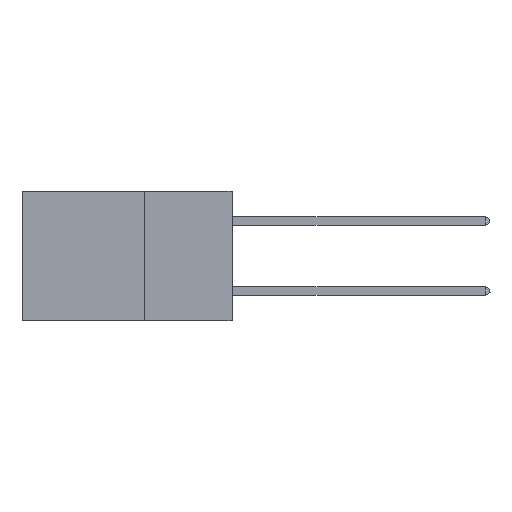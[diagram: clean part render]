
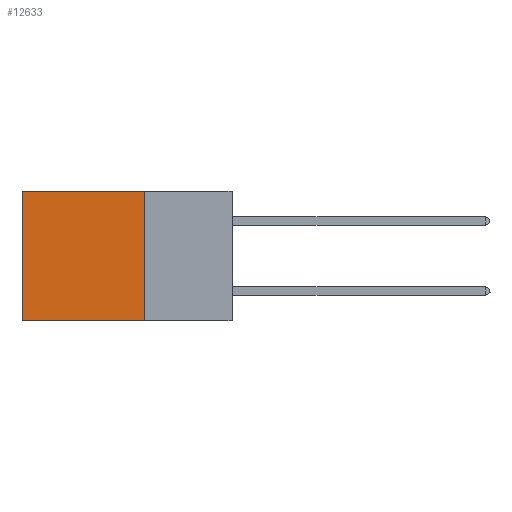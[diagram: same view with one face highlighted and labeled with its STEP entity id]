
A CAD part, left-side view. The second image highlights one B-rep face of the part: STEP entity #12633.
In plain terms, the highlighted planar face has unit normal (-1, 0, 0).
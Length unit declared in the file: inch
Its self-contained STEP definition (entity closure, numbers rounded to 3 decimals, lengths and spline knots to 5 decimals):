
#1057 = CARTESIAN_POINT ( 'NONE',  ( 0.2875, 0.25, 0. ) ) ;
#1160 = CARTESIAN_POINT ( 'NONE',  ( 0.2875, 0.6, -0.37 ) ) ;
#1495 = PLANE ( 'NONE',  #9630 ) ;
#3088 = CARTESIAN_POINT ( 'NONE',  ( 0.2875, 0.25, 0. ) ) ;
#3526 = CARTESIAN_POINT ( 'NONE',  ( 0.2875, 0.25, 0. ) ) ;
#3814 = CARTESIAN_POINT ( 'NONE',  ( 0.2875, 0.25, -0.37 ) ) ;
#4068 = VECTOR ( 'NONE', #19564, 39.37008 ) ;
#5462 = DIRECTION ( 'NONE',  ( 1., 0., 0. ) ) ;
#5641 = ORIENTED_EDGE ( 'NONE', *, *, #22986, .F. ) ;
#5736 = LINE ( 'NONE', #3814, #12072 ) ;
#8291 = CARTESIAN_POINT ( 'NONE',  ( 0.2875, 0.6, 0. ) ) ;
#9358 = EDGE_LOOP ( 'NONE', ( #25087, #5641, #19317, #11969 ) ) ;
#9630 = AXIS2_PLACEMENT_3D ( 'NONE', #3526, #5462, #24938 ) ;
#10706 = LINE ( 'NONE', #3088, #4068 ) ;
#11969 = ORIENTED_EDGE ( 'NONE', *, *, #16224, .T. ) ;
#12072 = VECTOR ( 'NONE', #18723, 39.37008 ) ;
#12633 = ADVANCED_FACE ( 'NONE', ( #27156 ), #1495, .F. ) ;
#12864 = EDGE_CURVE ( 'NONE', #13849, #25302, #15051, .T. ) ;
#13849 = VERTEX_POINT ( 'NONE', #19700 ) ;
#14086 = VECTOR ( 'NONE', #19574, 39.37008 ) ;
#15051 = LINE ( 'NONE', #1057, #14086 ) ;
#15396 = VECTOR ( 'NONE', #19002, 39.37008 ) ;
#16224 = EDGE_CURVE ( 'NONE', #13849, #17164, #10706, .T. ) ;
#17061 = LINE ( 'NONE', #8291, #15396 ) ;
#17164 = VERTEX_POINT ( 'NONE', #20154 ) ;
#18723 = DIRECTION ( 'NONE',  ( 0., 1., 0. ) ) ;
#19002 = DIRECTION ( 'NONE',  ( 0., 0., -1. ) ) ;
#19317 = ORIENTED_EDGE ( 'NONE', *, *, #12864, .F. ) ;
#19564 = DIRECTION ( 'NONE',  ( 0., 1., 0. ) ) ;
#19574 = DIRECTION ( 'NONE',  ( 0., 0., -1. ) ) ;
#19700 = CARTESIAN_POINT ( 'NONE',  ( 0.2875, 0.25, 0. ) ) ;
#20154 = CARTESIAN_POINT ( 'NONE',  ( 0.2875, 0.6, 0. ) ) ;
#22986 = EDGE_CURVE ( 'NONE', #25302, #23207, #5736, .T. ) ;
#23207 = VERTEX_POINT ( 'NONE', #1160 ) ;
#23547 = EDGE_CURVE ( 'NONE', #17164, #23207, #17061, .T. ) ;
#24938 = DIRECTION ( 'NONE',  ( 0., 0., -1. ) ) ;
#25087 = ORIENTED_EDGE ( 'NONE', *, *, #23547, .T. ) ;
#25302 = VERTEX_POINT ( 'NONE', #26240 ) ;
#26240 = CARTESIAN_POINT ( 'NONE',  ( 0.2875, 0.25, -0.37 ) ) ;
#27156 = FACE_OUTER_BOUND ( 'NONE', #9358, .T. ) ;
